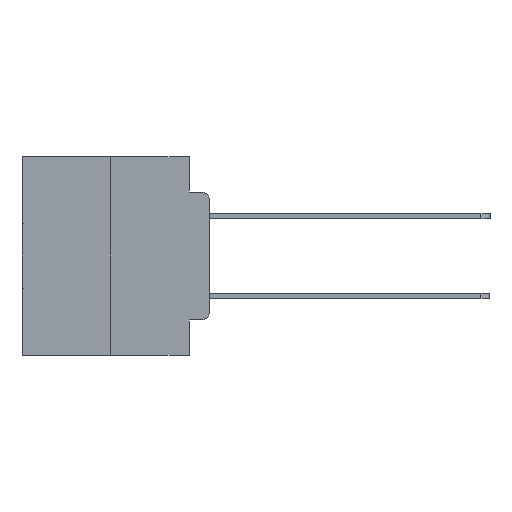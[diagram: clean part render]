
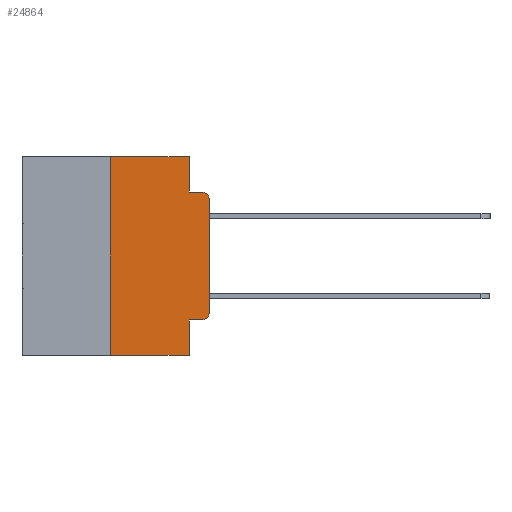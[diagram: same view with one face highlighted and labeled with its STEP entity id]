
A CAD part, left-side view. The second image highlights one B-rep face of the part: STEP entity #24864.
In plain terms, the highlighted planar face has unit normal (-1, 0, 0).
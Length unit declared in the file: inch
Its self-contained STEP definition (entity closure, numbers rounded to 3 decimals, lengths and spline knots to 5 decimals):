
#72 = ORIENTED_EDGE ( 'NONE', *, *, #20686, .T. ) ;
#1223 = LINE ( 'NONE', #16895, #29465 ) ;
#1279 = VECTOR ( 'NONE', #24800, 39.37008 ) ;
#1585 = ORIENTED_EDGE ( 'NONE', *, *, #13108, .T. ) ;
#2756 = CIRCLE ( 'NONE', #3911, 0.02 ) ;
#2765 = PLANE ( 'NONE',  #11409 ) ;
#3214 = EDGE_CURVE ( 'NONE', #9764, #24697, #12185, .T. ) ;
#3253 = DIRECTION ( 'NONE',  ( -1., 0., 0. ) ) ;
#3732 = CARTESIAN_POINT ( 'NONE',  ( 0., 0.473, -0.5 ) ) ;
#3911 = AXIS2_PLACEMENT_3D ( 'NONE', #17204, #3253, #19465 ) ;
#4532 = CARTESIAN_POINT ( 'NONE',  ( 0., 0.02, -0.1085 ) ) ;
#4758 = EDGE_CURVE ( 'NONE', #5454, #6576, #14999, .T. ) ;
#4920 = CARTESIAN_POINT ( 'NONE',  ( 0., 0., -0.3915 ) ) ;
#5454 = VERTEX_POINT ( 'NONE', #8731 ) ;
#6041 = EDGE_CURVE ( 'NONE', #20880, #28406, #9804, .T. ) ;
#6576 = VERTEX_POINT ( 'NONE', #23111 ) ;
#6719 = ORIENTED_EDGE ( 'NONE', *, *, #18650, .F. ) ;
#6864 = DIRECTION ( 'NONE',  ( 0., 0., -1. ) ) ;
#7184 = LINE ( 'NONE', #8899, #18774 ) ;
#8053 = CARTESIAN_POINT ( 'NONE',  ( 0., 0.051, 0. ) ) ;
#8101 = VERTEX_POINT ( 'NONE', #17396 ) ;
#8307 = LINE ( 'NONE', #11207, #1279 ) ;
#8731 = CARTESIAN_POINT ( 'NONE',  ( 0., 0.25, -0.5 ) ) ;
#8877 = VECTOR ( 'NONE', #11104, 39.37008 ) ;
#8899 = CARTESIAN_POINT ( 'NONE',  ( 0., 0.051, 0. ) ) ;
#9764 = VERTEX_POINT ( 'NONE', #29187 ) ;
#9804 = LINE ( 'NONE', #23414, #11637 ) ;
#9858 = CARTESIAN_POINT ( 'NONE',  ( 0., 0.473, 0. ) ) ;
#10266 = VECTOR ( 'NONE', #10422, 39.37008 ) ;
#10422 = DIRECTION ( 'NONE',  ( 0., 0., -1. ) ) ;
#11104 = DIRECTION ( 'NONE',  ( 0., 0., 1. ) ) ;
#11207 = CARTESIAN_POINT ( 'NONE',  ( 0., 0.051, -0.4115 ) ) ;
#11369 = AXIS2_PLACEMENT_3D ( 'NONE', #4532, #20653, #6864 ) ;
#11409 = AXIS2_PLACEMENT_3D ( 'NONE', #9858, #25699, #12223 ) ;
#11637 = VECTOR ( 'NONE', #14541, 39.37008 ) ;
#12019 = DIRECTION ( 'NONE',  ( 0., -1., 0. ) ) ;
#12185 = LINE ( 'NONE', #27753, #24164 ) ;
#12223 = DIRECTION ( 'NONE',  ( 0., 0., -1. ) ) ;
#12244 = ORIENTED_EDGE ( 'NONE', *, *, #22575, .T. ) ;
#12657 = EDGE_LOOP ( 'NONE', ( #16920, #12244, #18330, #6719, #13716, #26329, #21125, #16578, #72, #1585 ) ) ;
#13108 = EDGE_CURVE ( 'NONE', #16074, #20880, #2756, .T. ) ;
#13532 = VERTEX_POINT ( 'NONE', #13953 ) ;
#13707 = DIRECTION ( 'NONE',  ( 0., 0., -1. ) ) ;
#13716 = ORIENTED_EDGE ( 'NONE', *, *, #3214, .F. ) ;
#13953 = CARTESIAN_POINT ( 'NONE',  ( 0., 0.02, -0.0885 ) ) ;
#14299 = VERTEX_POINT ( 'NONE', #27940 ) ;
#14541 = DIRECTION ( 'NONE',  ( 0., 0., 1. ) ) ;
#14999 = LINE ( 'NONE', #3732, #27554 ) ;
#15719 = FACE_OUTER_BOUND ( 'NONE', #12657, .T. ) ;
#16074 = VERTEX_POINT ( 'NONE', #18136 ) ;
#16441 = LINE ( 'NONE', #8053, #10266 ) ;
#16578 = ORIENTED_EDGE ( 'NONE', *, *, #26630, .F. ) ;
#16895 = CARTESIAN_POINT ( 'NONE',  ( 0., 0.051, -0.0885 ) ) ;
#16920 = ORIENTED_EDGE ( 'NONE', *, *, #6041, .T. ) ;
#17204 = CARTESIAN_POINT ( 'NONE',  ( 0., 0.02, -0.3915 ) ) ;
#17396 = CARTESIAN_POINT ( 'NONE',  ( 0., 0.051, -0.0885 ) ) ;
#18136 = CARTESIAN_POINT ( 'NONE',  ( 0., 0.02, -0.4115 ) ) ;
#18330 = ORIENTED_EDGE ( 'NONE', *, *, #21628, .F. ) ;
#18650 = EDGE_CURVE ( 'NONE', #24697, #8101, #16441, .T. ) ;
#18774 = VECTOR ( 'NONE', #13707, 39.37008 ) ;
#19465 = DIRECTION ( 'NONE',  ( 0., 0., -1. ) ) ;
#19909 = DIRECTION ( 'NONE',  ( 0., -1., 0. ) ) ;
#20653 = DIRECTION ( 'NONE',  ( -1., 0., 0. ) ) ;
#20686 = EDGE_CURVE ( 'NONE', #14299, #16074, #8307, .T. ) ;
#20764 = CARTESIAN_POINT ( 'NONE',  ( 0., 0.051, 0. ) ) ;
#20880 = VERTEX_POINT ( 'NONE', #4920 ) ;
#21125 = ORIENTED_EDGE ( 'NONE', *, *, #4758, .T. ) ;
#21628 = EDGE_CURVE ( 'NONE', #8101, #13532, #1223, .T. ) ;
#22520 = CIRCLE ( 'NONE', #11369, 0.02 ) ;
#22575 = EDGE_CURVE ( 'NONE', #28406, #13532, #22520, .T. ) ;
#23111 = CARTESIAN_POINT ( 'NONE',  ( 0., 0.051, -0.5 ) ) ;
#23414 = CARTESIAN_POINT ( 'NONE',  ( 0., 0., 0. ) ) ;
#24164 = VECTOR ( 'NONE', #12019, 39.37008 ) ;
#24697 = VERTEX_POINT ( 'NONE', #20764 ) ;
#24800 = DIRECTION ( 'NONE',  ( 0., -1., 0. ) ) ;
#24864 = ADVANCED_FACE ( 'NONE', ( #15719 ), #2765, .F. ) ;
#25699 = DIRECTION ( 'NONE',  ( 1., 0., 0. ) ) ;
#26329 = ORIENTED_EDGE ( 'NONE', *, *, #29607, .F. ) ;
#26630 = EDGE_CURVE ( 'NONE', #14299, #6576, #7184, .T. ) ;
#26865 = CARTESIAN_POINT ( 'NONE',  ( 0., 0.25, 0. ) ) ;
#27554 = VECTOR ( 'NONE', #19909, 39.37008 ) ;
#27753 = CARTESIAN_POINT ( 'NONE',  ( 0., 0.473, 0. ) ) ;
#27940 = CARTESIAN_POINT ( 'NONE',  ( 0., 0.051, -0.4115 ) ) ;
#28082 = DIRECTION ( 'NONE',  ( 0., -1., 0. ) ) ;
#28353 = LINE ( 'NONE', #26865, #8877 ) ;
#28406 = VERTEX_POINT ( 'NONE', #29248 ) ;
#29187 = CARTESIAN_POINT ( 'NONE',  ( 0., 0.25, 0. ) ) ;
#29248 = CARTESIAN_POINT ( 'NONE',  ( 0., 0., -0.1085 ) ) ;
#29465 = VECTOR ( 'NONE', #28082, 39.37008 ) ;
#29607 = EDGE_CURVE ( 'NONE', #5454, #9764, #28353, .T. ) ;
